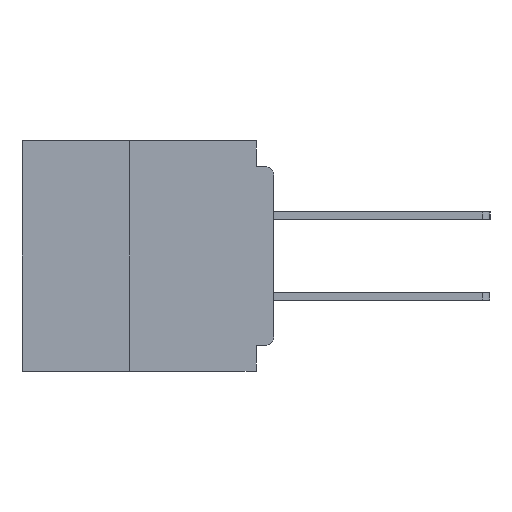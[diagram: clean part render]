
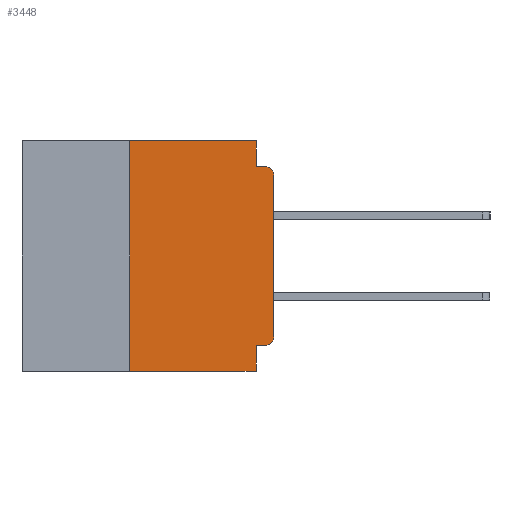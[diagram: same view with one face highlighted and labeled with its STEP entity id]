
A CAD part, left-side view. The second image highlights one B-rep face of the part: STEP entity #3448.
In plain terms, the highlighted planar face has unit normal (-1, 0, 0).
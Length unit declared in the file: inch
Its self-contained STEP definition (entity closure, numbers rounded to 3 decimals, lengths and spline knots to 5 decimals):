
#886 = CARTESIAN_POINT ( 'NONE',  ( 0., 0., -0.34 ) ) ;
#1154 = DIRECTION ( 'NONE',  ( 0., -1., 0. ) ) ;
#1917 = VERTEX_POINT ( 'NONE', #886 ) ;
#2073 = VERTEX_POINT ( 'NONE', #27864 ) ;
#2132 = DIRECTION ( 'NONE',  ( 0., 0., 1. ) ) ;
#2827 = LINE ( 'NONE', #32838, #30943 ) ;
#2845 = ORIENTED_EDGE ( 'NONE', *, *, #46249, .F. ) ;
#3276 = EDGE_CURVE ( 'NONE', #2073, #1917, #9838, .T. ) ;
#3448 = ADVANCED_FACE ( 'NONE', ( #65123 ), #37885, .F. ) ;
#5708 = VECTOR ( 'NONE', #54482, 39.37008 ) ;
#6473 = LINE ( 'NONE', #42333, #18937 ) ;
#7026 = DIRECTION ( 'NONE',  ( 0., 1., 0. ) ) ;
#7819 = CARTESIAN_POINT ( 'NONE',  ( 0., 0.031, 0. ) ) ;
#8875 = DIRECTION ( 'NONE',  ( 0., 0., 1. ) ) ;
#9372 = ORIENTED_EDGE ( 'NONE', *, *, #21040, .F. ) ;
#9774 = AXIS2_PLACEMENT_3D ( 'NONE', #48244, #43168, #11559 ) ;
#9838 = CIRCLE ( 'NONE', #35875, 0.015 ) ;
#9958 = ORIENTED_EDGE ( 'NONE', *, *, #44931, .T. ) ;
#10692 = EDGE_CURVE ( 'NONE', #57336, #31633, #25770, .T. ) ;
#10922 = ORIENTED_EDGE ( 'NONE', *, *, #10692, .F. ) ;
#11148 = VERTEX_POINT ( 'NONE', #54234 ) ;
#11559 = DIRECTION ( 'NONE',  ( 0., 0., -1. ) ) ;
#12731 = ORIENTED_EDGE ( 'NONE', *, *, #37766, .F. ) ;
#15508 = DIRECTION ( 'NONE',  ( -1., 0., 0. ) ) ;
#16030 = DIRECTION ( 'NONE',  ( 0., -1., 0. ) ) ;
#16083 = EDGE_CURVE ( 'NONE', #1917, #65178, #52734, .T. ) ;
#17461 = CARTESIAN_POINT ( 'NONE',  ( 0., 0.031, -0.4 ) ) ;
#17586 = CARTESIAN_POINT ( 'NONE',  ( 0., 0.015, -0.045 ) ) ;
#18421 = VECTOR ( 'NONE', #7026, 39.37008 ) ;
#18937 = VECTOR ( 'NONE', #16030, 39.37008 ) ;
#19681 = CARTESIAN_POINT ( 'NONE',  ( 0., 0., -0.06 ) ) ;
#19800 = LINE ( 'NONE', #33305, #5708 ) ;
#19819 = LINE ( 'NONE', #17461, #61882 ) ;
#21040 = EDGE_CURVE ( 'NONE', #36598, #57336, #2827, .T. ) ;
#22136 = CARTESIAN_POINT ( 'NONE',  ( 0., 0.015, -0.06 ) ) ;
#22474 = CARTESIAN_POINT ( 'NONE',  ( 0., 0.031, -0.4 ) ) ;
#24110 = VECTOR ( 'NONE', #50592, 39.37008 ) ;
#25770 = LINE ( 'NONE', #55904, #24110 ) ;
#27435 = DIRECTION ( 'NONE',  ( 0., 0., -1. ) ) ;
#27853 = EDGE_CURVE ( 'NONE', #59449, #56618, #6473, .T. ) ;
#27864 = CARTESIAN_POINT ( 'NONE',  ( 0., 0.015, -0.355 ) ) ;
#29546 = VECTOR ( 'NONE', #2132, 39.37008 ) ;
#29710 = ORIENTED_EDGE ( 'NONE', *, *, #36000, .F. ) ;
#30943 = VECTOR ( 'NONE', #1154, 39.37008 ) ;
#31633 = VERTEX_POINT ( 'NONE', #52083 ) ;
#32838 = CARTESIAN_POINT ( 'NONE',  ( 0., 0.437, 0. ) ) ;
#33085 = CARTESIAN_POINT ( 'NONE',  ( 0., 0.25, 0. ) ) ;
#33305 = CARTESIAN_POINT ( 'NONE',  ( 0., 0., -0.045 ) ) ;
#33610 = CARTESIAN_POINT ( 'NONE',  ( 0., 0., -0.355 ) ) ;
#35875 = AXIS2_PLACEMENT_3D ( 'NONE', #47103, #15508, #52412 ) ;
#36000 = EDGE_CURVE ( 'NONE', #2073, #11148, #63829, .T. ) ;
#36598 = VERTEX_POINT ( 'NONE', #33085 ) ;
#37766 = EDGE_CURVE ( 'NONE', #11148, #56618, #19819, .T. ) ;
#37885 = PLANE ( 'NONE',  #9774 ) ;
#42333 = CARTESIAN_POINT ( 'NONE',  ( 0., 0.437, -0.4 ) ) ;
#43168 = DIRECTION ( 'NONE',  ( 1., 0., 0. ) ) ;
#44141 = CARTESIAN_POINT ( 'NONE',  ( 0., 0.25, -0.4 ) ) ;
#44358 = VERTEX_POINT ( 'NONE', #17586 ) ;
#44931 = EDGE_CURVE ( 'NONE', #65178, #44358, #48027, .T. ) ;
#46249 = EDGE_CURVE ( 'NONE', #31633, #44358, #19800, .T. ) ;
#47103 = CARTESIAN_POINT ( 'NONE',  ( 0., 0.015, -0.34 ) ) ;
#48027 = CIRCLE ( 'NONE', #52822, 0.015 ) ;
#48244 = CARTESIAN_POINT ( 'NONE',  ( 0., 0.437, 0. ) ) ;
#50592 = DIRECTION ( 'NONE',  ( 0., 0., -1. ) ) ;
#51057 = VECTOR ( 'NONE', #8875, 39.37008 ) ;
#51074 = CARTESIAN_POINT ( 'NONE',  ( 0., 0., 0. ) ) ;
#51935 = EDGE_LOOP ( 'NONE', ( #53238, #9958, #2845, #10922, #9372, #56301, #59923, #12731, #29710, #58177 ) ) ;
#52083 = CARTESIAN_POINT ( 'NONE',  ( 0., 0.031, -0.045 ) ) ;
#52412 = DIRECTION ( 'NONE',  ( 0., 0., -1. ) ) ;
#52734 = LINE ( 'NONE', #51074, #51057 ) ;
#52822 = AXIS2_PLACEMENT_3D ( 'NONE', #22136, #59025, #27435 ) ;
#53238 = ORIENTED_EDGE ( 'NONE', *, *, #16083, .T. ) ;
#54234 = CARTESIAN_POINT ( 'NONE',  ( 0., 0.031, -0.355 ) ) ;
#54482 = DIRECTION ( 'NONE',  ( 0., -1., 0. ) ) ;
#55904 = CARTESIAN_POINT ( 'NONE',  ( 0., 0.031, 0. ) ) ;
#56301 = ORIENTED_EDGE ( 'NONE', *, *, #59460, .F. ) ;
#56618 = VERTEX_POINT ( 'NONE', #22474 ) ;
#57336 = VERTEX_POINT ( 'NONE', #7819 ) ;
#57588 = LINE ( 'NONE', #60079, #29546 ) ;
#58177 = ORIENTED_EDGE ( 'NONE', *, *, #3276, .T. ) ;
#59025 = DIRECTION ( 'NONE',  ( -1., 0., 0. ) ) ;
#59449 = VERTEX_POINT ( 'NONE', #44141 ) ;
#59460 = EDGE_CURVE ( 'NONE', #59449, #36598, #57588, .T. ) ;
#59651 = DIRECTION ( 'NONE',  ( 0., 0., -1. ) ) ;
#59923 = ORIENTED_EDGE ( 'NONE', *, *, #27853, .T. ) ;
#60079 = CARTESIAN_POINT ( 'NONE',  ( 0., 0.25, -0.4 ) ) ;
#61882 = VECTOR ( 'NONE', #59651, 39.37008 ) ;
#63829 = LINE ( 'NONE', #33610, #18421 ) ;
#65123 = FACE_OUTER_BOUND ( 'NONE', #51935, .T. ) ;
#65178 = VERTEX_POINT ( 'NONE', #19681 ) ;
